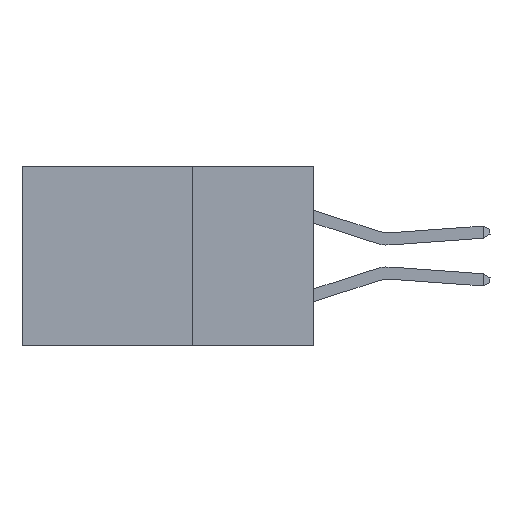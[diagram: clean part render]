
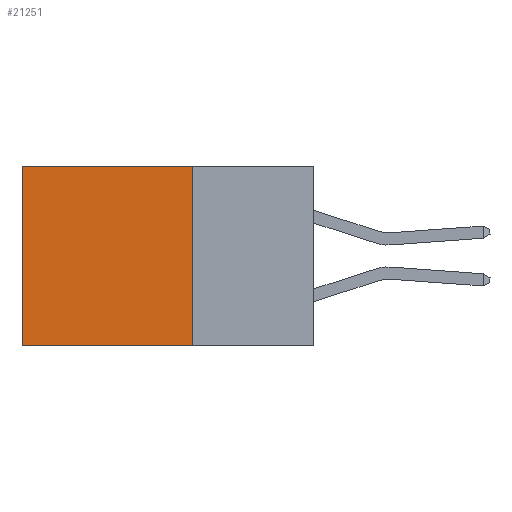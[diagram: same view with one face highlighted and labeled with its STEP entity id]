
A CAD part, left-side view. The second image highlights one B-rep face of the part: STEP entity #21251.
In plain terms, the highlighted planar face has unit normal (-1, 0, 0).
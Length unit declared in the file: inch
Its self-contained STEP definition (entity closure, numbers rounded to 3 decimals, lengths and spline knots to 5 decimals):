
#72 = ORIENTED_EDGE ( 'NONE', *, *, #18484, .T. ) ;
#220 = VERTEX_POINT ( 'NONE', #10879 ) ;
#266 = DIRECTION ( 'NONE',  ( 1., 0., 0. ) ) ;
#1524 = LINE ( 'NONE', #4404, #15072 ) ;
#2796 = AXIS2_PLACEMENT_3D ( 'NONE', #20570, #266, #15018 ) ;
#3407 = PLANE ( 'NONE',  #2796 ) ;
#3418 = ORIENTED_EDGE ( 'NONE', *, *, #14188, .F. ) ;
#4063 = CARTESIAN_POINT ( 'NONE',  ( 0.2875, 0.6, -0.37 ) ) ;
#4208 = FACE_OUTER_BOUND ( 'NONE', #13476, .T. ) ;
#4224 = ORIENTED_EDGE ( 'NONE', *, *, #6720, .T. ) ;
#4404 = CARTESIAN_POINT ( 'NONE',  ( 0.2875, 0.6, 0. ) ) ;
#5630 = DIRECTION ( 'NONE',  ( 0., 1., 0. ) ) ;
#6720 = EDGE_CURVE ( 'NONE', #220, #23496, #17021, .T. ) ;
#7495 = CARTESIAN_POINT ( 'NONE',  ( 0.2875, 0.25, -0.37 ) ) ;
#9042 = LINE ( 'NONE', #16318, #11347 ) ;
#9589 = CARTESIAN_POINT ( 'NONE',  ( 0.2875, 0.25, 0. ) ) ;
#10315 = DIRECTION ( 'NONE',  ( 0., 0., -1. ) ) ;
#10879 = CARTESIAN_POINT ( 'NONE',  ( 0.2875, 0.25, 0. ) ) ;
#11347 = VECTOR ( 'NONE', #23759, 39.37008 ) ;
#12480 = VERTEX_POINT ( 'NONE', #7495 ) ;
#12860 = CARTESIAN_POINT ( 'NONE',  ( 0.2875, 0.25, 0. ) ) ;
#13448 = VECTOR ( 'NONE', #17075, 39.37008 ) ;
#13476 = EDGE_LOOP ( 'NONE', ( #72, #17199, #3418, #4224 ) ) ;
#14188 = EDGE_CURVE ( 'NONE', #220, #12480, #18091, .T. ) ;
#15018 = DIRECTION ( 'NONE',  ( 0., 0., -1. ) ) ;
#15072 = VECTOR ( 'NONE', #10315, 39.37008 ) ;
#16318 = CARTESIAN_POINT ( 'NONE',  ( 0.2875, 0.25, -0.37 ) ) ;
#17021 = LINE ( 'NONE', #9589, #19055 ) ;
#17075 = DIRECTION ( 'NONE',  ( 0., 0., -1. ) ) ;
#17199 = ORIENTED_EDGE ( 'NONE', *, *, #23004, .F. ) ;
#18091 = LINE ( 'NONE', #12860, #13448 ) ;
#18484 = EDGE_CURVE ( 'NONE', #23496, #19519, #1524, .T. ) ;
#19055 = VECTOR ( 'NONE', #5630, 39.37008 ) ;
#19519 = VERTEX_POINT ( 'NONE', #4063 ) ;
#19940 = CARTESIAN_POINT ( 'NONE',  ( 0.2875, 0.6, 0. ) ) ;
#20570 = CARTESIAN_POINT ( 'NONE',  ( 0.2875, 0.25, 0. ) ) ;
#21251 = ADVANCED_FACE ( 'NONE', ( #4208 ), #3407, .F. ) ;
#23004 = EDGE_CURVE ( 'NONE', #12480, #19519, #9042, .T. ) ;
#23496 = VERTEX_POINT ( 'NONE', #19940 ) ;
#23759 = DIRECTION ( 'NONE',  ( 0., 1., 0. ) ) ;
